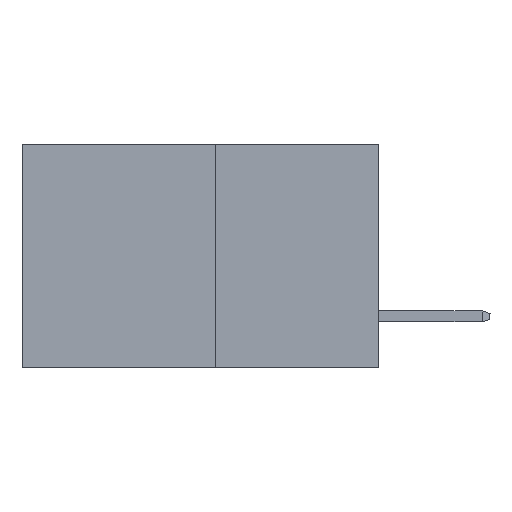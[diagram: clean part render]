
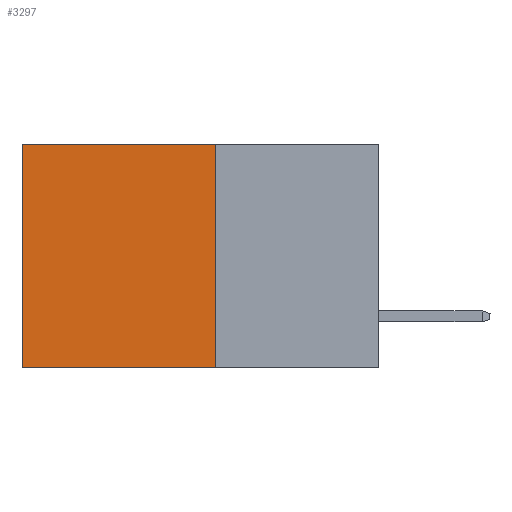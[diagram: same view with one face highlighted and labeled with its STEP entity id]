
A CAD part, left-side view. The second image highlights one B-rep face of the part: STEP entity #3297.
In plain terms, the highlighted planar face has unit normal (-1, 0, 0).
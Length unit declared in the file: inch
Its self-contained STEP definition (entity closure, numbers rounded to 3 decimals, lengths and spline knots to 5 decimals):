
#323 = LINE ( 'NONE', #3890, #8805 ) ;
#905 = EDGE_CURVE ( 'NONE', #4056, #5681, #2639, .T. ) ;
#912 = VERTEX_POINT ( 'NONE', #8729 ) ;
#1524 = EDGE_LOOP ( 'NONE', ( #6863, #6900, #6936, #7078 ) ) ;
#1955 = CARTESIAN_POINT ( 'NONE',  ( 0.277, 0.27, 0. ) ) ;
#2639 = LINE ( 'NONE', #9740, #6836 ) ;
#3223 = VECTOR ( 'NONE', #8810, 39.37008 ) ;
#3297 = ADVANCED_FACE ( 'NONE', ( #4862 ), #9034, .F. ) ;
#3433 = DIRECTION ( 'NONE',  ( 0., 0., -1. ) ) ;
#3498 = VERTEX_POINT ( 'NONE', #7781 ) ;
#3809 = DIRECTION ( 'NONE',  ( 0., 1., 0. ) ) ;
#3890 = CARTESIAN_POINT ( 'NONE',  ( 0.277, 0.27, -0.37 ) ) ;
#4056 = VERTEX_POINT ( 'NONE', #9133 ) ;
#4522 = EDGE_CURVE ( 'NONE', #912, #3498, #8459, .T. ) ;
#4716 = VECTOR ( 'NONE', #7660, 39.37008 ) ;
#4862 = FACE_OUTER_BOUND ( 'NONE', #1524, .T. ) ;
#4987 = EDGE_CURVE ( 'NONE', #3498, #5681, #323, .T. ) ;
#5343 = LINE ( 'NONE', #1955, #3223 ) ;
#5681 = VERTEX_POINT ( 'NONE', #8191 ) ;
#5909 = EDGE_CURVE ( 'NONE', #912, #4056, #5343, .T. ) ;
#6591 = CARTESIAN_POINT ( 'NONE',  ( 0.277, 0.27, -0.37 ) ) ;
#6836 = VECTOR ( 'NONE', #9665, 39.37008 ) ;
#6863 = ORIENTED_EDGE ( 'NONE', *, *, #905, .T. ) ;
#6900 = ORIENTED_EDGE ( 'NONE', *, *, #4987, .F. ) ;
#6936 = ORIENTED_EDGE ( 'NONE', *, *, #4522, .F. ) ;
#7078 = ORIENTED_EDGE ( 'NONE', *, *, #5909, .T. ) ;
#7587 = CARTESIAN_POINT ( 'NONE',  ( 0.277, 0.27, -0.37 ) ) ;
#7660 = DIRECTION ( 'NONE',  ( 0., 0., -1. ) ) ;
#7736 = DIRECTION ( 'NONE',  ( 1., 0., 0. ) ) ;
#7781 = CARTESIAN_POINT ( 'NONE',  ( 0.277, 0.27, -0.37 ) ) ;
#8191 = CARTESIAN_POINT ( 'NONE',  ( 0.277, 0.59, -0.37 ) ) ;
#8459 = LINE ( 'NONE', #7587, #4716 ) ;
#8729 = CARTESIAN_POINT ( 'NONE',  ( 0.277, 0.27, 0. ) ) ;
#8805 = VECTOR ( 'NONE', #3809, 39.37008 ) ;
#8810 = DIRECTION ( 'NONE',  ( 0., 1., 0. ) ) ;
#9034 = PLANE ( 'NONE',  #9759 ) ;
#9133 = CARTESIAN_POINT ( 'NONE',  ( 0.277, 0.59, 0. ) ) ;
#9665 = DIRECTION ( 'NONE',  ( 0., 0., -1. ) ) ;
#9740 = CARTESIAN_POINT ( 'NONE',  ( 0.277, 0.59, -0.37 ) ) ;
#9759 = AXIS2_PLACEMENT_3D ( 'NONE', #6591, #7736, #3433 ) ;
